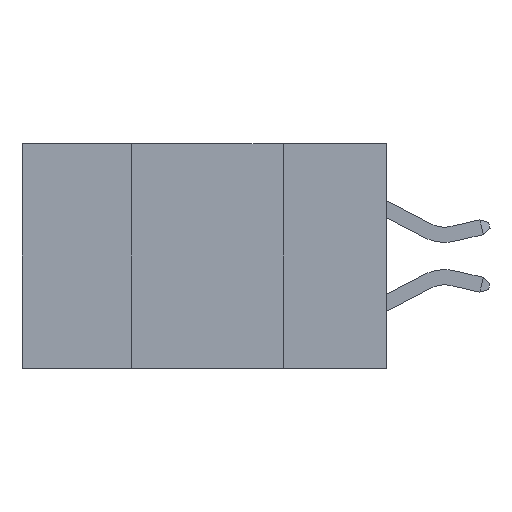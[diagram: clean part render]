
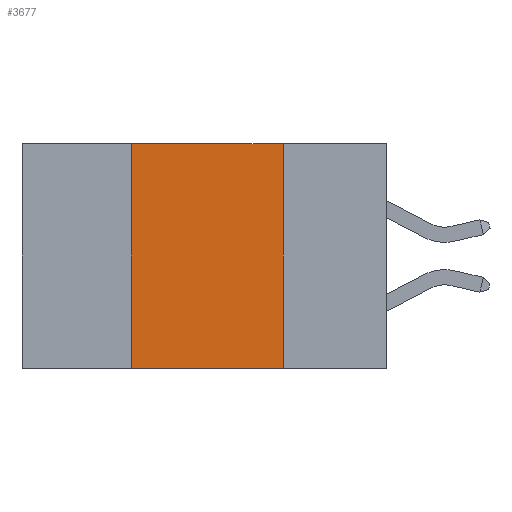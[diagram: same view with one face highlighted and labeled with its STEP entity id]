
A CAD part, left-side view. The second image highlights one B-rep face of the part: STEP entity #3677.
In plain terms, the highlighted planar face has unit normal (-1, 0, 0).
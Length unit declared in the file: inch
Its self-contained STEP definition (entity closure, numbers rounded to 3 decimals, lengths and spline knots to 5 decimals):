
#78 = VECTOR ( 'NONE', #14833, 39.37008 ) ;
#414 = ORIENTED_EDGE ( 'NONE', *, *, #12230, .F. ) ;
#464 = ORIENTED_EDGE ( 'NONE', *, *, #12413, .F. ) ;
#494 = DIRECTION ( 'NONE',  ( 0., -1., 0. ) ) ;
#692 = ORIENTED_EDGE ( 'NONE', *, *, #8618, .F. ) ;
#844 = ORIENTED_EDGE ( 'NONE', *, *, #16971, .T. ) ;
#967 = LINE ( 'NONE', #4219, #7732 ) ;
#1043 = VERTEX_POINT ( 'NONE', #14702 ) ;
#2615 = DIRECTION ( 'NONE',  ( 0., 0., -1. ) ) ;
#3386 = AXIS2_PLACEMENT_3D ( 'NONE', #9335, #10705, #2615 ) ;
#3624 = CARTESIAN_POINT ( 'NONE',  ( 0., 0.42, -0.37 ) ) ;
#3677 = ADVANCED_FACE ( 'NONE', ( #14529 ), #17269, .F. ) ;
#4219 = CARTESIAN_POINT ( 'NONE',  ( 0., 0.17, 0. ) ) ;
#4784 = VERTEX_POINT ( 'NONE', #3624 ) ;
#5597 = DIRECTION ( 'NONE',  ( 0., 0., -1. ) ) ;
#6530 = CARTESIAN_POINT ( 'NONE',  ( 0., 0.42, 0. ) ) ;
#7732 = VECTOR ( 'NONE', #5597, 39.37008 ) ;
#7880 = DIRECTION ( 'NONE',  ( 0., 0., 1. ) ) ;
#8339 = LINE ( 'NONE', #8566, #11517 ) ;
#8566 = CARTESIAN_POINT ( 'NONE',  ( 0., 0.6, 0. ) ) ;
#8618 = EDGE_CURVE ( 'NONE', #4784, #1043, #15339, .T. ) ;
#9250 = EDGE_LOOP ( 'NONE', ( #414, #464, #692, #844 ) ) ;
#9335 = CARTESIAN_POINT ( 'NONE',  ( 0., 0.6, 0. ) ) ;
#10705 = DIRECTION ( 'NONE',  ( 1., 0., 0. ) ) ;
#10847 = LINE ( 'NONE', #13547, #78 ) ;
#11517 = VECTOR ( 'NONE', #494, 39.37008 ) ;
#11575 = VERTEX_POINT ( 'NONE', #13363 ) ;
#12230 = EDGE_CURVE ( 'NONE', #11575, #16052, #967, .T. ) ;
#12413 = EDGE_CURVE ( 'NONE', #1043, #11575, #8339, .T. ) ;
#13363 = CARTESIAN_POINT ( 'NONE',  ( 0., 0.17, 0. ) ) ;
#13547 = CARTESIAN_POINT ( 'NONE',  ( 0., 0.6, -0.37 ) ) ;
#14529 = FACE_OUTER_BOUND ( 'NONE', #9250, .T. ) ;
#14702 = CARTESIAN_POINT ( 'NONE',  ( 0., 0.42, 0. ) ) ;
#14833 = DIRECTION ( 'NONE',  ( 0., -1., 0. ) ) ;
#14922 = VECTOR ( 'NONE', #7880, 39.37008 ) ;
#15339 = LINE ( 'NONE', #6530, #14922 ) ;
#16052 = VERTEX_POINT ( 'NONE', #17003 ) ;
#16971 = EDGE_CURVE ( 'NONE', #4784, #16052, #10847, .T. ) ;
#17003 = CARTESIAN_POINT ( 'NONE',  ( 0., 0.17, -0.37 ) ) ;
#17269 = PLANE ( 'NONE',  #3386 ) ;
